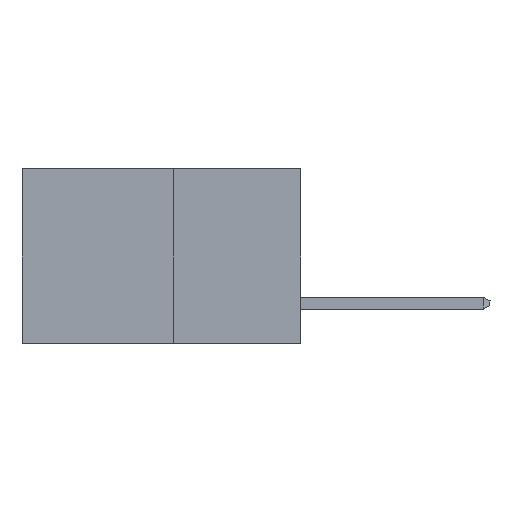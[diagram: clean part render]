
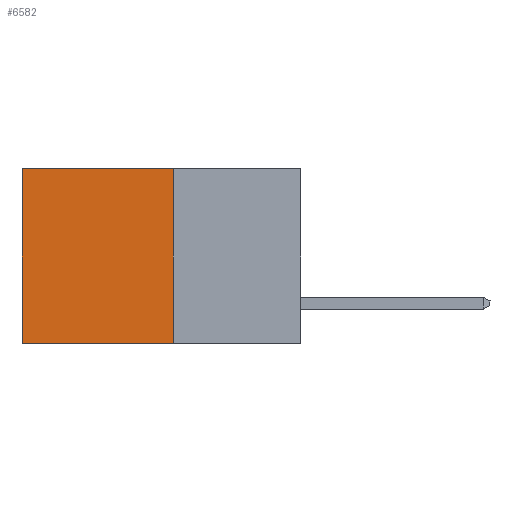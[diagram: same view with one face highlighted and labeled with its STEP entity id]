
A CAD part, left-side view. The second image highlights one B-rep face of the part: STEP entity #6582.
In plain terms, the highlighted planar face has unit normal (-1, 0, 0).
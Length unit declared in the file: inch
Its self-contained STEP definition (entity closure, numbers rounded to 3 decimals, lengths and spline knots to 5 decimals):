
#1 = CARTESIAN_POINT ( 'NONE',  ( 0.277, 0.27, -0.37 ) ) ;
#32 = VECTOR ( 'NONE', #4907, 39.37008 ) ;
#148 = VECTOR ( 'NONE', #4340, 39.37008 ) ;
#329 = PLANE ( 'NONE',  #3909 ) ;
#449 = VERTEX_POINT ( 'NONE', #5836 ) ;
#761 = EDGE_LOOP ( 'NONE', ( #8717, #7951, #6172, #3812 ) ) ;
#954 = VERTEX_POINT ( 'NONE', #6824 ) ;
#1098 = FACE_OUTER_BOUND ( 'NONE', #761, .T. ) ;
#1381 = VECTOR ( 'NONE', #3787, 39.37008 ) ;
#2440 = LINE ( 'NONE', #4351, #148 ) ;
#2757 = CARTESIAN_POINT ( 'NONE',  ( 0.277, 0.27, 0. ) ) ;
#3764 = CARTESIAN_POINT ( 'NONE',  ( 0.277, 0.27, -0.37 ) ) ;
#3787 = DIRECTION ( 'NONE',  ( 0., 0., -1. ) ) ;
#3812 = ORIENTED_EDGE ( 'NONE', *, *, #4460, .T. ) ;
#3909 = AXIS2_PLACEMENT_3D ( 'NONE', #1, #9980, #9851 ) ;
#3938 = VECTOR ( 'NONE', #5394, 39.37008 ) ;
#4340 = DIRECTION ( 'NONE',  ( 0., 0., -1. ) ) ;
#4351 = CARTESIAN_POINT ( 'NONE',  ( 0.277, 0.59, -0.37 ) ) ;
#4460 = EDGE_CURVE ( 'NONE', #6707, #954, #4684, .T. ) ;
#4684 = LINE ( 'NONE', #2757, #32 ) ;
#4907 = DIRECTION ( 'NONE',  ( 0., 1., 0. ) ) ;
#5313 = VERTEX_POINT ( 'NONE', #9681 ) ;
#5394 = DIRECTION ( 'NONE',  ( 0., 1., 0. ) ) ;
#5421 = CARTESIAN_POINT ( 'NONE',  ( 0.277, 0.27, -0.37 ) ) ;
#5794 = EDGE_CURVE ( 'NONE', #449, #5313, #5931, .T. ) ;
#5836 = CARTESIAN_POINT ( 'NONE',  ( 0.277, 0.27, -0.37 ) ) ;
#5857 = CARTESIAN_POINT ( 'NONE',  ( 0.277, 0.27, 0. ) ) ;
#5931 = LINE ( 'NONE', #5421, #3938 ) ;
#5970 = EDGE_CURVE ( 'NONE', #954, #5313, #2440, .T. ) ;
#6069 = EDGE_CURVE ( 'NONE', #6707, #449, #7602, .T. ) ;
#6172 = ORIENTED_EDGE ( 'NONE', *, *, #6069, .F. ) ;
#6582 = ADVANCED_FACE ( 'NONE', ( #1098 ), #329, .F. ) ;
#6707 = VERTEX_POINT ( 'NONE', #5857 ) ;
#6824 = CARTESIAN_POINT ( 'NONE',  ( 0.277, 0.59, 0. ) ) ;
#7602 = LINE ( 'NONE', #3764, #1381 ) ;
#7951 = ORIENTED_EDGE ( 'NONE', *, *, #5794, .F. ) ;
#8717 = ORIENTED_EDGE ( 'NONE', *, *, #5970, .T. ) ;
#9681 = CARTESIAN_POINT ( 'NONE',  ( 0.277, 0.59, -0.37 ) ) ;
#9851 = DIRECTION ( 'NONE',  ( 0., 0., -1. ) ) ;
#9980 = DIRECTION ( 'NONE',  ( 1., 0., 0. ) ) ;
